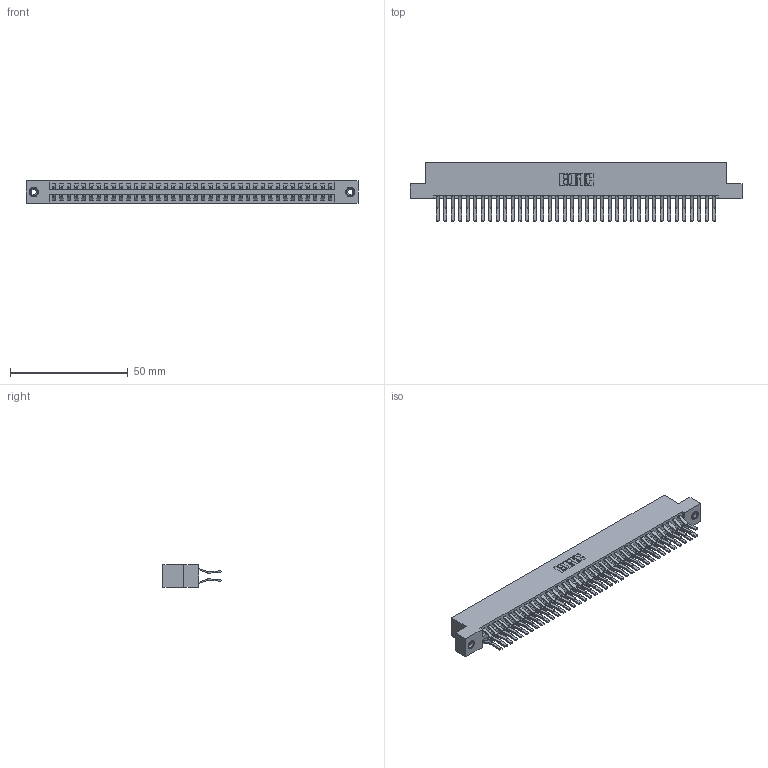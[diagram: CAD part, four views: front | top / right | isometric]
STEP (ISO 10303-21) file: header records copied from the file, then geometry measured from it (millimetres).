
FILE_DESCRIPTION (( 'STEP AP203' ), '1' );
FILE_NAME ('396-076-560-208.STEP', '2018-09-09T14:49:54', ( '' ), ( '' ), 'SwSTEP 2.0', 'SolidWorks 2016', '' );
FILE_SCHEMA (( 'CONFIG_CONTROL_DESIGN' ));
Length unit declared in the file: inch
Products named in the file (4): 346 Part_Flush Mounting Lugs - 0.156 Dia-TI; 345-292-001_560 Tail; 345-250-001_345-250-003-102; 396-076-560-208
Assembly tree (79 placements, depth 2):
  396-076-560-208
    346 Part_Flush Mounting Lugs - 0.156 Dia-TI
    345-292-001_560 Tail  x76
    345-250-001_345-250-003-102  x2
Bounding box: 141.22 x 24.78 x 9.4 mm (x, y, z)
Volume: 14231.7 mm3; surface area: 20848.6 mm2
Topology: 79 solids, 79 shells, 4286 faces, 12701 edges, 8358 vertices
Faces by surface type: plane 2768, cylinder 1502, cone 12, torus 4
Entity records: 26612 total; most frequent: CARTESIAN_POINT 4375, ORIENTED_EDGE 4302, DIRECTION 3937, EDGE_CURVE 2151, VECTOR 1843, LINE 1843, VERTEX_POINT 1428, AXIS2_PLACEMENT_3D 1047
